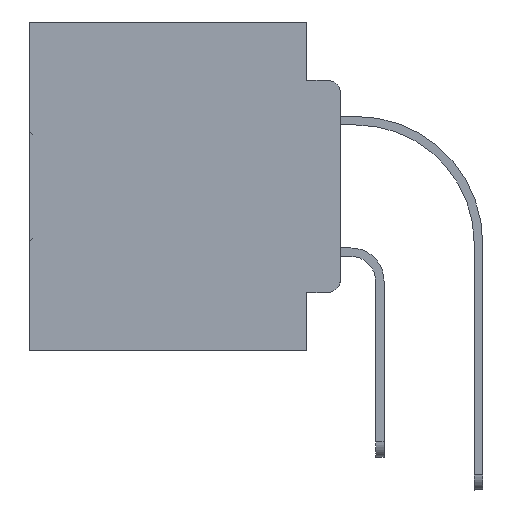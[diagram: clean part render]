
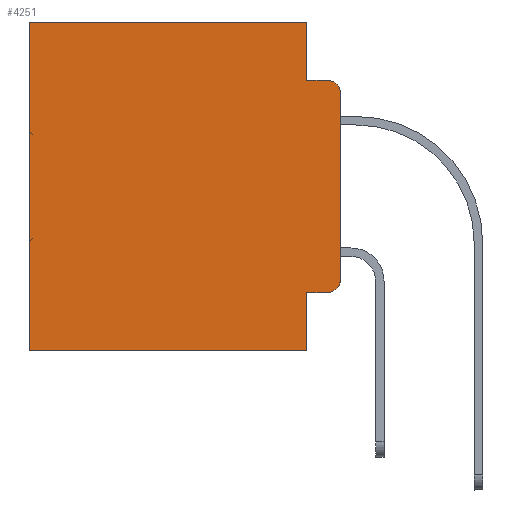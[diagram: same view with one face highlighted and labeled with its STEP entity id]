
A CAD part, left-side view. The second image highlights one B-rep face of the part: STEP entity #4251.
In plain terms, the highlighted planar face has unit normal (-1, 0, 0).
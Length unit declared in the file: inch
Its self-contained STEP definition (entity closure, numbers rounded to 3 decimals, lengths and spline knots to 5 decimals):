
#125 = DIRECTION ( 'NONE',  ( 0., 0., -1. ) ) ;
#417 = CARTESIAN_POINT ( 'NONE',  ( 0.298, 0.051, -0.5 ) ) ;
#749 = CARTESIAN_POINT ( 'NONE',  ( 0.298, 0.473, -0.5 ) ) ;
#817 = CARTESIAN_POINT ( 'NONE',  ( 0.298, 0.051, 0. ) ) ;
#1233 = EDGE_CURVE ( 'NONE', #9585, #24100, #7478, .T. ) ;
#1377 = EDGE_CURVE ( 'NONE', #27223, #28064, #27634, .T. ) ;
#1640 = CARTESIAN_POINT ( 'NONE',  ( 0.298, 0., -0.3915 ) ) ;
#1950 = EDGE_CURVE ( 'NONE', #35272, #5536, #11604, .T. ) ;
#2231 = DIRECTION ( 'NONE',  ( 0., 0., -1. ) ) ;
#3140 = ORIENTED_EDGE ( 'NONE', *, *, #32052, .F. ) ;
#3894 = VECTOR ( 'NONE', #125, 39.37008 ) ;
#3934 = LINE ( 'NONE', #18743, #15203 ) ;
#4096 = ORIENTED_EDGE ( 'NONE', *, *, #10602, .F. ) ;
#4251 = ADVANCED_FACE ( 'NONE', ( #9524 ), #35174, .F. ) ;
#4468 = DIRECTION ( 'NONE',  ( 0., 1., 0. ) ) ;
#4505 = ORIENTED_EDGE ( 'NONE', *, *, #34466, .F. ) ;
#4721 = DIRECTION ( 'NONE',  ( 0., -1., 0. ) ) ;
#5536 = VERTEX_POINT ( 'NONE', #417 ) ;
#5555 = ORIENTED_EDGE ( 'NONE', *, *, #35089, .T. ) ;
#5949 = CIRCLE ( 'NONE', #10617, 0.02 ) ;
#7100 = DIRECTION ( 'NONE',  ( 0., 0., -1. ) ) ;
#7478 = LINE ( 'NONE', #18646, #12060 ) ;
#7663 = LINE ( 'NONE', #29844, #22544 ) ;
#8014 = CARTESIAN_POINT ( 'NONE',  ( 0.298, 0.051, 0. ) ) ;
#8492 = DIRECTION ( 'NONE',  ( 0., 0., -1. ) ) ;
#9152 = LINE ( 'NONE', #10201, #26348 ) ;
#9294 = AXIS2_PLACEMENT_3D ( 'NONE', #12245, #18483, #15550 ) ;
#9524 = FACE_OUTER_BOUND ( 'NONE', #28487, .T. ) ;
#9585 = VERTEX_POINT ( 'NONE', #33769 ) ;
#9931 = CARTESIAN_POINT ( 'NONE',  ( 0.298, 0.02, -0.3915 ) ) ;
#10182 = EDGE_CURVE ( 'NONE', #27223, #9585, #9152, .T. ) ;
#10201 = CARTESIAN_POINT ( 'NONE',  ( 0.298, 0., 0. ) ) ;
#10584 = VECTOR ( 'NONE', #7100, 39.37008 ) ;
#10594 = CARTESIAN_POINT ( 'NONE',  ( 0.298, 0.051, -0.4115 ) ) ;
#10602 = EDGE_CURVE ( 'NONE', #5536, #24100, #3934, .T. ) ;
#10617 = AXIS2_PLACEMENT_3D ( 'NONE', #27560, #18943, #8492 ) ;
#10859 = VECTOR ( 'NONE', #22636, 39.37008 ) ;
#11604 = LINE ( 'NONE', #817, #10859 ) ;
#12060 = VECTOR ( 'NONE', #24170, 39.37008 ) ;
#12159 = CARTESIAN_POINT ( 'NONE',  ( 0.298, 0.02, -0.0885 ) ) ;
#12245 = CARTESIAN_POINT ( 'NONE',  ( 0.298, 0., 0. ) ) ;
#12579 = CARTESIAN_POINT ( 'NONE',  ( 0.298, 0., 0. ) ) ;
#13279 = DIRECTION ( 'NONE',  ( 0., 1., 0. ) ) ;
#15203 = VECTOR ( 'NONE', #4468, 39.37008 ) ;
#15550 = DIRECTION ( 'NONE',  ( 0., 0., -1. ) ) ;
#16109 = ORIENTED_EDGE ( 'NONE', *, *, #1950, .F. ) ;
#16148 = CARTESIAN_POINT ( 'NONE',  ( 0.298, 0., -0.1085 ) ) ;
#16903 = CARTESIAN_POINT ( 'NONE',  ( 0.298, 0.051, -0.4115 ) ) ;
#17867 = CARTESIAN_POINT ( 'NONE',  ( 0.298, 0.051, 0. ) ) ;
#17992 = LINE ( 'NONE', #10594, #27047 ) ;
#18483 = DIRECTION ( 'NONE',  ( 1., 0., 0. ) ) ;
#18646 = CARTESIAN_POINT ( 'NONE',  ( 0.298, 0.473, 0. ) ) ;
#18743 = CARTESIAN_POINT ( 'NONE',  ( 0.298, 0., -0.5 ) ) ;
#18943 = DIRECTION ( 'NONE',  ( -1., 0., 0. ) ) ;
#19544 = ORIENTED_EDGE ( 'NONE', *, *, #1233, .T. ) ;
#21002 = VERTEX_POINT ( 'NONE', #12159 ) ;
#21120 = DIRECTION ( 'NONE',  ( -1., 0., 0. ) ) ;
#21303 = CARTESIAN_POINT ( 'NONE',  ( 0.298, 0.02, -0.4115 ) ) ;
#22437 = EDGE_CURVE ( 'NONE', #26057, #34027, #33181, .T. ) ;
#22544 = VECTOR ( 'NONE', #4721, 39.37008 ) ;
#22636 = DIRECTION ( 'NONE',  ( 0., 0., -1. ) ) ;
#24100 = VERTEX_POINT ( 'NONE', #749 ) ;
#24143 = LINE ( 'NONE', #12579, #10584 ) ;
#24170 = DIRECTION ( 'NONE',  ( 0., 0., -1. ) ) ;
#26057 = VERTEX_POINT ( 'NONE', #21303 ) ;
#26108 = ORIENTED_EDGE ( 'NONE', *, *, #35421, .T. ) ;
#26348 = VECTOR ( 'NONE', #13279, 39.37008 ) ;
#27047 = VECTOR ( 'NONE', #29186, 39.37008 ) ;
#27223 = VERTEX_POINT ( 'NONE', #17867 ) ;
#27560 = CARTESIAN_POINT ( 'NONE',  ( 0.298, 0.02, -0.1085 ) ) ;
#27634 = LINE ( 'NONE', #8014, #3894 ) ;
#28064 = VERTEX_POINT ( 'NONE', #34251 ) ;
#28487 = EDGE_LOOP ( 'NONE', ( #4505, #5555, #3140, #33688, #29943, #19544, #4096, #16109, #26108, #34516 ) ) ;
#29067 = VERTEX_POINT ( 'NONE', #16148 ) ;
#29186 = DIRECTION ( 'NONE',  ( 0., -1., 0. ) ) ;
#29844 = CARTESIAN_POINT ( 'NONE',  ( 0.298, 0.051, -0.0885 ) ) ;
#29943 = ORIENTED_EDGE ( 'NONE', *, *, #10182, .T. ) ;
#31440 = AXIS2_PLACEMENT_3D ( 'NONE', #9931, #21120, #2231 ) ;
#32052 = EDGE_CURVE ( 'NONE', #28064, #21002, #7663, .T. ) ;
#33181 = CIRCLE ( 'NONE', #31440, 0.02 ) ;
#33688 = ORIENTED_EDGE ( 'NONE', *, *, #1377, .F. ) ;
#33769 = CARTESIAN_POINT ( 'NONE',  ( 0.298, 0.473, 0. ) ) ;
#34027 = VERTEX_POINT ( 'NONE', #1640 ) ;
#34251 = CARTESIAN_POINT ( 'NONE',  ( 0.298, 0.051, -0.0885 ) ) ;
#34466 = EDGE_CURVE ( 'NONE', #29067, #34027, #24143, .T. ) ;
#34516 = ORIENTED_EDGE ( 'NONE', *, *, #22437, .T. ) ;
#35089 = EDGE_CURVE ( 'NONE', #29067, #21002, #5949, .T. ) ;
#35174 = PLANE ( 'NONE',  #9294 ) ;
#35272 = VERTEX_POINT ( 'NONE', #16903 ) ;
#35421 = EDGE_CURVE ( 'NONE', #35272, #26057, #17992, .T. ) ;
